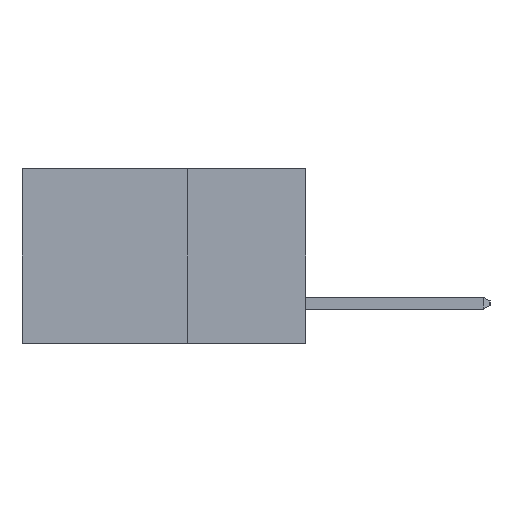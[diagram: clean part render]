
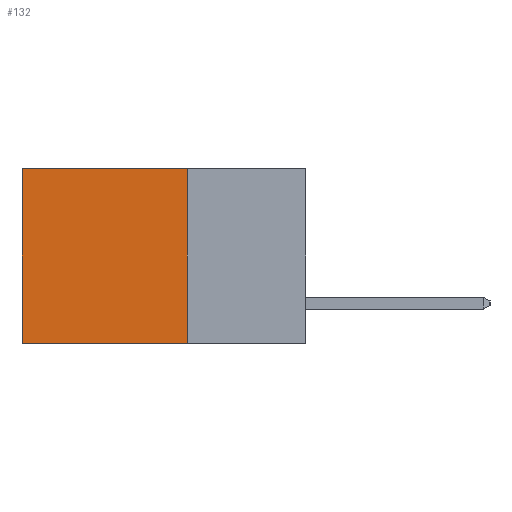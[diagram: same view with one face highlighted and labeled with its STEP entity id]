
A CAD part, left-side view. The second image highlights one B-rep face of the part: STEP entity #132.
In plain terms, the highlighted planar face has unit normal (-1, 0, 0).
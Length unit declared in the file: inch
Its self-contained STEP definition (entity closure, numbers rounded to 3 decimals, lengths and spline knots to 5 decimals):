
#132 = ADVANCED_FACE ( 'NONE', ( #16404 ), #5041, .F. ) ;
#762 = LINE ( 'NONE', #3549, #8088 ) ;
#1158 = VECTOR ( 'NONE', #6583, 39.37008 ) ;
#2315 = EDGE_CURVE ( 'NONE', #13818, #3769, #762, .T. ) ;
#2393 = EDGE_LOOP ( 'NONE', ( #3616, #17204, #14541, #14032 ) ) ;
#2593 = LINE ( 'NONE', #14747, #16700 ) ;
#3159 = EDGE_CURVE ( 'NONE', #15792, #3769, #12504, .T. ) ;
#3549 = CARTESIAN_POINT ( 'NONE',  ( 0.298, 0.6, 0. ) ) ;
#3616 = ORIENTED_EDGE ( 'NONE', *, *, #2315, .T. ) ;
#3769 = VERTEX_POINT ( 'NONE', #12256 ) ;
#3787 = DIRECTION ( 'NONE',  ( 0., 1., 0. ) ) ;
#4462 = CARTESIAN_POINT ( 'NONE',  ( 0.298, 0.6, 0. ) ) ;
#4739 = VECTOR ( 'NONE', #6016, 39.37008 ) ;
#4741 = EDGE_CURVE ( 'NONE', #14674, #15792, #12027, .T. ) ;
#5041 = PLANE ( 'NONE',  #14403 ) ;
#5200 = CARTESIAN_POINT ( 'NONE',  ( 0.298, 0.25, -0.37 ) ) ;
#6016 = DIRECTION ( 'NONE',  ( 0., 0., -1. ) ) ;
#6583 = DIRECTION ( 'NONE',  ( 0., 1., 0. ) ) ;
#8088 = VECTOR ( 'NONE', #14502, 39.37008 ) ;
#8835 = CARTESIAN_POINT ( 'NONE',  ( 0.298, 0.25, 0. ) ) ;
#8885 = DIRECTION ( 'NONE',  ( 0., 0., -1. ) ) ;
#9958 = EDGE_CURVE ( 'NONE', #14674, #13818, #2593, .T. ) ;
#12027 = LINE ( 'NONE', #12828, #4739 ) ;
#12256 = CARTESIAN_POINT ( 'NONE',  ( 0.298, 0.6, -0.37 ) ) ;
#12504 = LINE ( 'NONE', #5200, #1158 ) ;
#12828 = CARTESIAN_POINT ( 'NONE',  ( 0.298, 0.25, 0. ) ) ;
#13110 = DIRECTION ( 'NONE',  ( 1., 0., 0. ) ) ;
#13818 = VERTEX_POINT ( 'NONE', #4462 ) ;
#13988 = CARTESIAN_POINT ( 'NONE',  ( 0.298, 0.25, -0.37 ) ) ;
#14032 = ORIENTED_EDGE ( 'NONE', *, *, #9958, .T. ) ;
#14403 = AXIS2_PLACEMENT_3D ( 'NONE', #16355, #13110, #8885 ) ;
#14502 = DIRECTION ( 'NONE',  ( 0., 0., -1. ) ) ;
#14541 = ORIENTED_EDGE ( 'NONE', *, *, #4741, .F. ) ;
#14674 = VERTEX_POINT ( 'NONE', #8835 ) ;
#14747 = CARTESIAN_POINT ( 'NONE',  ( 0.298, 0.25, 0. ) ) ;
#15792 = VERTEX_POINT ( 'NONE', #13988 ) ;
#16355 = CARTESIAN_POINT ( 'NONE',  ( 0.298, 0.25, 0. ) ) ;
#16404 = FACE_OUTER_BOUND ( 'NONE', #2393, .T. ) ;
#16700 = VECTOR ( 'NONE', #3787, 39.37008 ) ;
#17204 = ORIENTED_EDGE ( 'NONE', *, *, #3159, .F. ) ;
